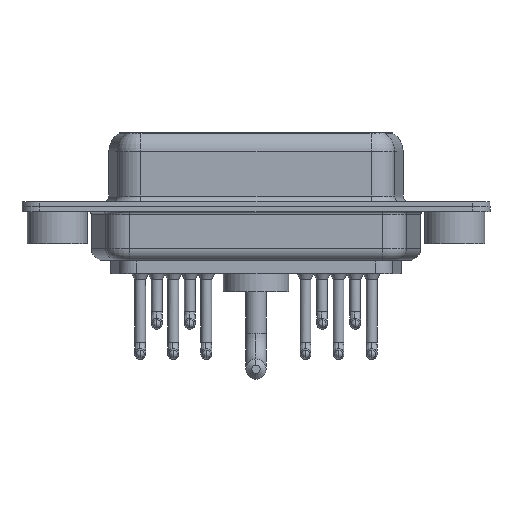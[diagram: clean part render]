
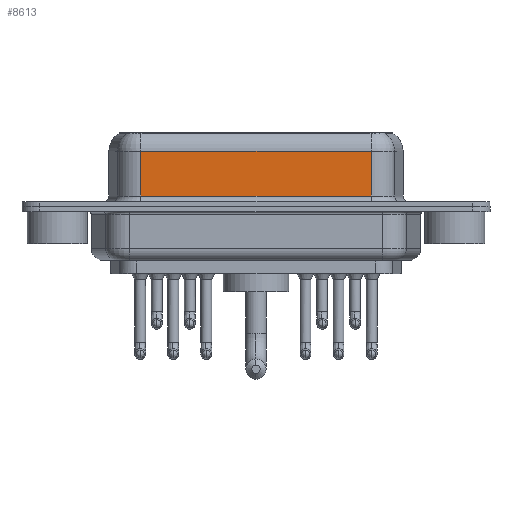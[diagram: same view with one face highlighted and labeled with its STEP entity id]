
A CAD part, front view. The second image highlights one B-rep face of the part: STEP entity #8613.
In plain terms, the highlighted planar face has unit normal (0, -1, 0).
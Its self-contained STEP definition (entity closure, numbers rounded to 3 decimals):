
#421 = ORIENTED_EDGE ( 'NONE', *, *, #14513, .T. ) ;
#558 = DIRECTION ( 'NONE',  ( 0., 0., 1. ) ) ;
#1355 = AXIS2_PLACEMENT_3D ( 'NONE', #3392, #10459, #558 ) ;
#2224 = VECTOR ( 'NONE', #11360, 1000. ) ;
#3355 = EDGE_CURVE ( 'NONE', #9367, #8616, #15772, .T. ) ;
#3392 = CARTESIAN_POINT ( 'NONE',  ( 26.287, -3.95, 6.4 ) ) ;
#4805 = FACE_OUTER_BOUND ( 'NONE', #6971, .T. ) ;
#5079 = VECTOR ( 'NONE', #13037, 1000. ) ;
#5522 = CARTESIAN_POINT ( 'NONE',  ( 26.287, -3.95, 6.4 ) ) ;
#6301 = CARTESIAN_POINT ( 'NONE',  ( 26.287, -3.95, 0.9 ) ) ;
#6971 = EDGE_LOOP ( 'NONE', ( #8434, #421, #12553, #16901 ) ) ;
#6997 = VERTEX_POINT ( 'NONE', #14122 ) ;
#7694 = EDGE_CURVE ( 'NONE', #15711, #8616, #11635, .T. ) ;
#8434 = ORIENTED_EDGE ( 'NONE', *, *, #3355, .F. ) ;
#8445 = DIRECTION ( 'NONE',  ( 0., 0., -1. ) ) ;
#8613 = ADVANCED_FACE ( 'NONE', ( #4805 ), #16307, .F. ) ;
#8616 = VERTEX_POINT ( 'NONE', #6301 ) ;
#9046 = CARTESIAN_POINT ( 'NONE',  ( 26.287, -3.95, 4.65 ) ) ;
#9317 = VECTOR ( 'NONE', #16317, 1000. ) ;
#9336 = EDGE_CURVE ( 'NONE', #6997, #15711, #9876, .T. ) ;
#9367 = VERTEX_POINT ( 'NONE', #18478 ) ;
#9876 = LINE ( 'NONE', #17143, #17335 ) ;
#10459 = DIRECTION ( 'NONE',  ( 0., 1., 0. ) ) ;
#11360 = DIRECTION ( 'NONE',  ( 1., 0., 0. ) ) ;
#11635 = LINE ( 'NONE', #12957, #2224 ) ;
#12553 = ORIENTED_EDGE ( 'NONE', *, *, #9336, .T. ) ;
#12957 = CARTESIAN_POINT ( 'NONE',  ( 26.287, -3.95, 0.9 ) ) ;
#13037 = DIRECTION ( 'NONE',  ( 0., 0., -1. ) ) ;
#14122 = CARTESIAN_POINT ( 'NONE',  ( 7.013, -3.95, 4.65 ) ) ;
#14149 = LINE ( 'NONE', #9046, #9317 ) ;
#14513 = EDGE_CURVE ( 'NONE', #9367, #6997, #14149, .T. ) ;
#15711 = VERTEX_POINT ( 'NONE', #16711 ) ;
#15772 = LINE ( 'NONE', #5522, #5079 ) ;
#16307 = PLANE ( 'NONE',  #1355 ) ;
#16317 = DIRECTION ( 'NONE',  ( -1., 0., 0. ) ) ;
#16711 = CARTESIAN_POINT ( 'NONE',  ( 7.013, -3.95, 0.9 ) ) ;
#16901 = ORIENTED_EDGE ( 'NONE', *, *, #7694, .T. ) ;
#17143 = CARTESIAN_POINT ( 'NONE',  ( 7.013, -3.95, 6.4 ) ) ;
#17335 = VECTOR ( 'NONE', #8445, 1000. ) ;
#18478 = CARTESIAN_POINT ( 'NONE',  ( 26.287, -3.95, 4.65 ) ) ;
